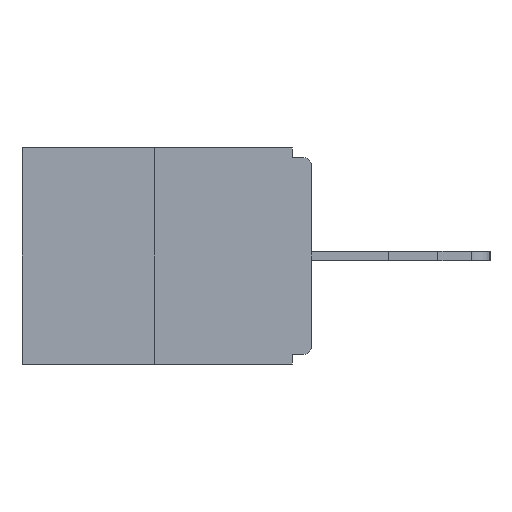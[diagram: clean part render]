
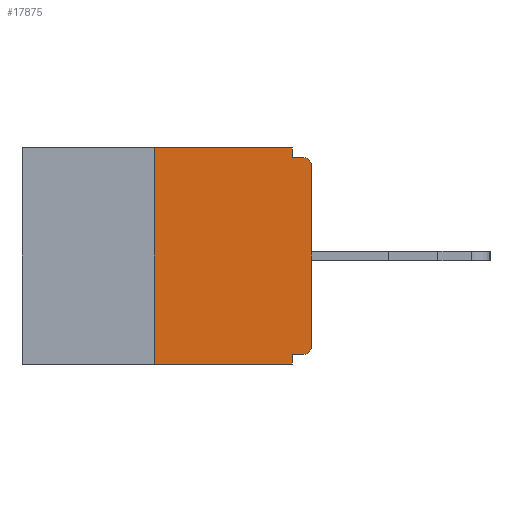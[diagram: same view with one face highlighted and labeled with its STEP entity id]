
A CAD part, left-side view. The second image highlights one B-rep face of the part: STEP entity #17875.
In plain terms, the highlighted planar face has unit normal (-1, 0, 0).
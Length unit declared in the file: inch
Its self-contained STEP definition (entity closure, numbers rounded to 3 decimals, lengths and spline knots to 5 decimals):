
#98 = ORIENTED_EDGE ( 'NONE', *, *, #27091, .F. ) ;
#332 = DIRECTION ( 'NONE',  ( 0., -1., 0. ) ) ;
#734 = LINE ( 'NONE', #2844, #21218 ) ;
#1105 = DIRECTION ( 'NONE',  ( 0., 0., -1. ) ) ;
#1420 = LINE ( 'NONE', #26781, #22545 ) ;
#1537 = ORIENTED_EDGE ( 'NONE', *, *, #22093, .F. ) ;
#2052 = LINE ( 'NONE', #14768, #25655 ) ;
#2711 = ORIENTED_EDGE ( 'NONE', *, *, #9965, .F. ) ;
#2844 = CARTESIAN_POINT ( 'NONE',  ( 0., 0., -0.328 ) ) ;
#3208 = DIRECTION ( 'NONE',  ( -1., 0., 0. ) ) ;
#3865 = PLANE ( 'NONE',  #27503 ) ;
#4585 = ORIENTED_EDGE ( 'NONE', *, *, #26570, .T. ) ;
#4734 = AXIS2_PLACEMENT_3D ( 'NONE', #4871, #21952, #22100 ) ;
#4851 = VERTEX_POINT ( 'NONE', #27636 ) ;
#4871 = CARTESIAN_POINT ( 'NONE',  ( 0., 0.015, -0.03 ) ) ;
#5299 = VECTOR ( 'NONE', #5697, 39.37008 ) ;
#5697 = DIRECTION ( 'NONE',  ( 0., 0., -1. ) ) ;
#5797 = CARTESIAN_POINT ( 'NONE',  ( 0., 0.015, -0.328 ) ) ;
#5822 = CIRCLE ( 'NONE', #9395, 0.015 ) ;
#6007 = CARTESIAN_POINT ( 'NONE',  ( 0., 0.031, -0.015 ) ) ;
#6406 = VECTOR ( 'NONE', #10329, 39.37008 ) ;
#6996 = EDGE_CURVE ( 'NONE', #23901, #11659, #734, .T. ) ;
#7017 = EDGE_CURVE ( 'NONE', #13061, #24871, #7944, .T. ) ;
#7675 = CARTESIAN_POINT ( 'NONE',  ( 0., 0.031, 0. ) ) ;
#7776 = LINE ( 'NONE', #16322, #5299 ) ;
#7944 = LINE ( 'NONE', #7675, #13608 ) ;
#7996 = VERTEX_POINT ( 'NONE', #14277 ) ;
#8278 = DIRECTION ( 'NONE',  ( 0., -1., 0. ) ) ;
#9395 = AXIS2_PLACEMENT_3D ( 'NONE', #11599, #3208, #1105 ) ;
#9431 = CARTESIAN_POINT ( 'NONE',  ( 0., 0.46, 0. ) ) ;
#9965 = EDGE_CURVE ( 'NONE', #11659, #19779, #7776, .T. ) ;
#10329 = DIRECTION ( 'NONE',  ( 0., -1., 0. ) ) ;
#10498 = CARTESIAN_POINT ( 'NONE',  ( 0., 0.031, -0.328 ) ) ;
#11562 = EDGE_CURVE ( 'NONE', #4851, #13061, #22204, .T. ) ;
#11599 = CARTESIAN_POINT ( 'NONE',  ( 0., 0.015, -0.313 ) ) ;
#11619 = VECTOR ( 'NONE', #8278, 39.37008 ) ;
#11659 = VERTEX_POINT ( 'NONE', #10498 ) ;
#12001 = EDGE_CURVE ( 'NONE', #23901, #26977, #5822, .T. ) ;
#12929 = FACE_OUTER_BOUND ( 'NONE', #25700, .T. ) ;
#13061 = VERTEX_POINT ( 'NONE', #16971 ) ;
#13608 = VECTOR ( 'NONE', #24919, 39.37008 ) ;
#14061 = ORIENTED_EDGE ( 'NONE', *, *, #12001, .T. ) ;
#14277 = CARTESIAN_POINT ( 'NONE',  ( 0., 0.015, -0.015 ) ) ;
#14768 = CARTESIAN_POINT ( 'NONE',  ( 0., 0., 0. ) ) ;
#14919 = DIRECTION ( 'NONE',  ( 0., 0., 1. ) ) ;
#15244 = EDGE_CURVE ( 'NONE', #16379, #19779, #17202, .T. ) ;
#15385 = ORIENTED_EDGE ( 'NONE', *, *, #7017, .F. ) ;
#15707 = ORIENTED_EDGE ( 'NONE', *, *, #11562, .F. ) ;
#15757 = CARTESIAN_POINT ( 'NONE',  ( 0., 0.25, -0.343 ) ) ;
#16119 = ORIENTED_EDGE ( 'NONE', *, *, #18806, .T. ) ;
#16322 = CARTESIAN_POINT ( 'NONE',  ( 0., 0.031, -0.343 ) ) ;
#16379 = VERTEX_POINT ( 'NONE', #15757 ) ;
#16971 = CARTESIAN_POINT ( 'NONE',  ( 0., 0.031, 0. ) ) ;
#17202 = LINE ( 'NONE', #23096, #6406 ) ;
#17235 = CIRCLE ( 'NONE', #4734, 0.015 ) ;
#17875 = ADVANCED_FACE ( 'NONE', ( #12929 ), #3865, .F. ) ;
#17902 = VERTEX_POINT ( 'NONE', #27532 ) ;
#18729 = ORIENTED_EDGE ( 'NONE', *, *, #6996, .F. ) ;
#18806 = EDGE_CURVE ( 'NONE', #17902, #7996, #17235, .T. ) ;
#19113 = DIRECTION ( 'NONE',  ( 1., 0., 0. ) ) ;
#19217 = VECTOR ( 'NONE', #332, 39.37008 ) ;
#19779 = VERTEX_POINT ( 'NONE', #22525 ) ;
#20865 = DIRECTION ( 'NONE',  ( 0., 1., 0. ) ) ;
#21218 = VECTOR ( 'NONE', #20865, 39.37008 ) ;
#21314 = CARTESIAN_POINT ( 'NONE',  ( 0., 0., -0.015 ) ) ;
#21354 = DIRECTION ( 'NONE',  ( 0., 0., -1. ) ) ;
#21952 = DIRECTION ( 'NONE',  ( -1., 0., 0. ) ) ;
#22093 = EDGE_CURVE ( 'NONE', #24871, #7996, #27490, .T. ) ;
#22100 = DIRECTION ( 'NONE',  ( 0., 0., -1. ) ) ;
#22204 = LINE ( 'NONE', #9431, #19217 ) ;
#22525 = CARTESIAN_POINT ( 'NONE',  ( 0., 0.031, -0.343 ) ) ;
#22545 = VECTOR ( 'NONE', #27197, 39.37008 ) ;
#23096 = CARTESIAN_POINT ( 'NONE',  ( 0., 0.46, -0.343 ) ) ;
#23172 = CARTESIAN_POINT ( 'NONE',  ( 0., 0., -0.313 ) ) ;
#23180 = CARTESIAN_POINT ( 'NONE',  ( 0., 0.46, 0. ) ) ;
#23901 = VERTEX_POINT ( 'NONE', #5797 ) ;
#24871 = VERTEX_POINT ( 'NONE', #6007 ) ;
#24919 = DIRECTION ( 'NONE',  ( 0., 0., -1. ) ) ;
#25655 = VECTOR ( 'NONE', #14919, 39.37008 ) ;
#25700 = EDGE_LOOP ( 'NONE', ( #15707, #98, #26045, #2711, #18729, #14061, #4585, #16119, #1537, #15385 ) ) ;
#26045 = ORIENTED_EDGE ( 'NONE', *, *, #15244, .T. ) ;
#26570 = EDGE_CURVE ( 'NONE', #26977, #17902, #2052, .T. ) ;
#26781 = CARTESIAN_POINT ( 'NONE',  ( 0., 0.25, 0. ) ) ;
#26977 = VERTEX_POINT ( 'NONE', #23172 ) ;
#27091 = EDGE_CURVE ( 'NONE', #16379, #4851, #1420, .T. ) ;
#27197 = DIRECTION ( 'NONE',  ( 0., 0., 1. ) ) ;
#27490 = LINE ( 'NONE', #21314, #11619 ) ;
#27503 = AXIS2_PLACEMENT_3D ( 'NONE', #23180, #19113, #21354 ) ;
#27532 = CARTESIAN_POINT ( 'NONE',  ( 0., 0., -0.03 ) ) ;
#27636 = CARTESIAN_POINT ( 'NONE',  ( 0., 0.25, 0. ) ) ;
